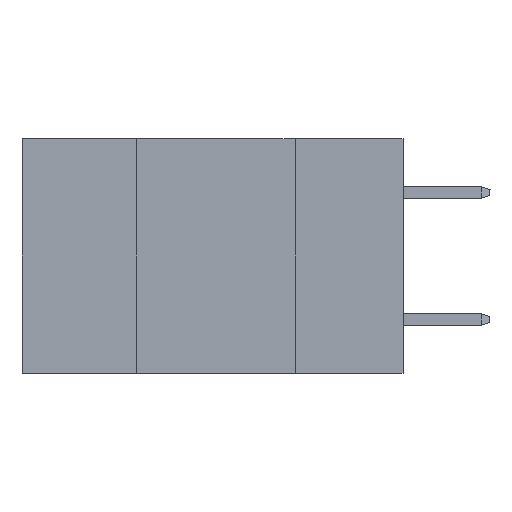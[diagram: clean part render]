
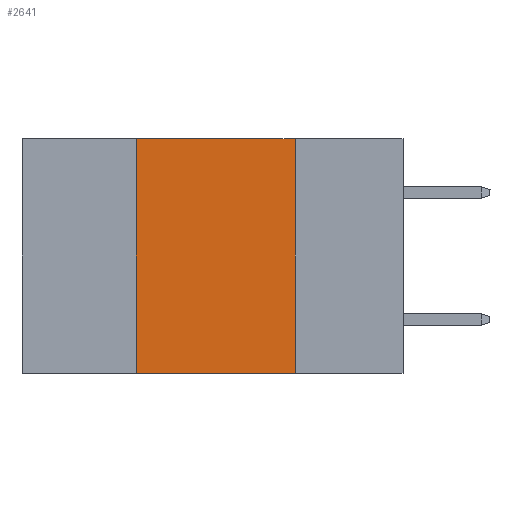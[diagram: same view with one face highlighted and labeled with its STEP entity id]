
A CAD part, left-side view. The second image highlights one B-rep face of the part: STEP entity #2641.
In plain terms, the highlighted planar face has unit normal (-1, 0, 0).
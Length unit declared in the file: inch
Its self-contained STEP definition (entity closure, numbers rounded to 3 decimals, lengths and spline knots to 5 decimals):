
#813 = ORIENTED_EDGE ( 'NONE', *, *, #1900, .F. ) ;
#827 = ORIENTED_EDGE ( 'NONE', *, *, #5524, .F. ) ;
#1785 = AXIS2_PLACEMENT_3D ( 'NONE', #4582, #15091, #8165 ) ;
#1900 = EDGE_CURVE ( 'NONE', #13383, #11016, #5015, .T. ) ;
#2641 = ADVANCED_FACE ( 'NONE', ( #4700 ), #20285, .F. ) ;
#3414 = CARTESIAN_POINT ( 'NONE',  ( 0., 0.42, 0. ) ) ;
#4582 = CARTESIAN_POINT ( 'NONE',  ( 0., 0.6, 0. ) ) ;
#4665 = VERTEX_POINT ( 'NONE', #3414 ) ;
#4685 = VECTOR ( 'NONE', #12049, 39.37008 ) ;
#4700 = FACE_OUTER_BOUND ( 'NONE', #11497, .T. ) ;
#5015 = LINE ( 'NONE', #5237, #4685 ) ;
#5237 = CARTESIAN_POINT ( 'NONE',  ( 0., 0.17, 0. ) ) ;
#5304 = CARTESIAN_POINT ( 'NONE',  ( 0., 0.42, 0. ) ) ;
#5524 = EDGE_CURVE ( 'NONE', #7263, #4665, #8788, .T. ) ;
#5929 = CARTESIAN_POINT ( 'NONE',  ( 0., 0.17, -0.37 ) ) ;
#7263 = VERTEX_POINT ( 'NONE', #21515 ) ;
#7374 = VECTOR ( 'NONE', #21973, 39.37008 ) ;
#7484 = EDGE_CURVE ( 'NONE', #7263, #11016, #22314, .T. ) ;
#8124 = VECTOR ( 'NONE', #19185, 39.37008 ) ;
#8165 = DIRECTION ( 'NONE',  ( 0., 0., -1. ) ) ;
#8189 = CARTESIAN_POINT ( 'NONE',  ( 0., 0.6, 0. ) ) ;
#8402 = VECTOR ( 'NONE', #18723, 39.37008 ) ;
#8788 = LINE ( 'NONE', #5304, #8124 ) ;
#9820 = LINE ( 'NONE', #8189, #8402 ) ;
#11016 = VERTEX_POINT ( 'NONE', #5929 ) ;
#11497 = EDGE_LOOP ( 'NONE', ( #813, #14428, #827, #19078 ) ) ;
#12049 = DIRECTION ( 'NONE',  ( 0., 0., -1. ) ) ;
#13383 = VERTEX_POINT ( 'NONE', #17185 ) ;
#14428 = ORIENTED_EDGE ( 'NONE', *, *, #17232, .F. ) ;
#15091 = DIRECTION ( 'NONE',  ( 1., 0., 0. ) ) ;
#16785 = CARTESIAN_POINT ( 'NONE',  ( 0., 0.6, -0.37 ) ) ;
#17185 = CARTESIAN_POINT ( 'NONE',  ( 0., 0.17, 0. ) ) ;
#17232 = EDGE_CURVE ( 'NONE', #4665, #13383, #9820, .T. ) ;
#18723 = DIRECTION ( 'NONE',  ( 0., -1., 0. ) ) ;
#19078 = ORIENTED_EDGE ( 'NONE', *, *, #7484, .T. ) ;
#19185 = DIRECTION ( 'NONE',  ( 0., 0., 1. ) ) ;
#20285 = PLANE ( 'NONE',  #1785 ) ;
#21515 = CARTESIAN_POINT ( 'NONE',  ( 0., 0.42, -0.37 ) ) ;
#21973 = DIRECTION ( 'NONE',  ( 0., -1., 0. ) ) ;
#22314 = LINE ( 'NONE', #16785, #7374 ) ;
